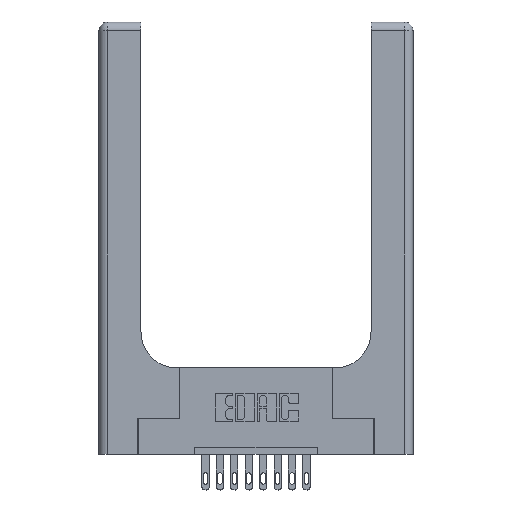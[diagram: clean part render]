
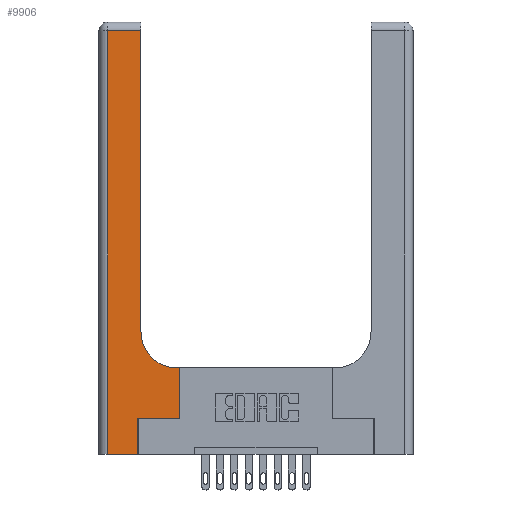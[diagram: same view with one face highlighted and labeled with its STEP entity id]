
A CAD part, top view. The second image highlights one B-rep face of the part: STEP entity #9906.
In plain terms, the highlighted planar face has unit normal (0, 0, 1).
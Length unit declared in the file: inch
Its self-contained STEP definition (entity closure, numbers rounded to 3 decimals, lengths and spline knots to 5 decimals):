
#43 = DIRECTION ( 'NONE',  ( 1., 0., 0. ) ) ;
#279 = LINE ( 'NONE', #14353, #12806 ) ;
#327 = LINE ( 'NONE', #10637, #10549 ) ;
#335 = CARTESIAN_POINT ( 'NONE',  ( 0.269, 0., 0.37 ) ) ;
#378 = CARTESIAN_POINT ( 'NONE',  ( 0.2915, 3., 0.37 ) ) ;
#451 = AXIS2_PLACEMENT_3D ( 'NONE', #11654, #6696, #12667 ) ;
#1412 = ORIENTED_EDGE ( 'NONE', *, *, #4250, .T. ) ;
#1574 = VECTOR ( 'NONE', #10758, 39.37008 ) ;
#1740 = AXIS2_PLACEMENT_3D ( 'NONE', #13222, #12018, #9772 ) ;
#1998 = VERTEX_POINT ( 'NONE', #11737 ) ;
#2088 = CARTESIAN_POINT ( 'NONE',  ( 0.5585, 0.25, 0.37 ) ) ;
#2108 = DIRECTION ( 'NONE',  ( -1., 0., 0. ) ) ;
#2135 = ORIENTED_EDGE ( 'NONE', *, *, #12017, .T. ) ;
#2408 = VERTEX_POINT ( 'NONE', #10790 ) ;
#2549 = FACE_OUTER_BOUND ( 'NONE', #7298, .T. ) ;
#2567 = VERTEX_POINT ( 'NONE', #14894 ) ;
#3411 = DIRECTION ( 'NONE',  ( 1., 0., 0. ) ) ;
#3450 = ORIENTED_EDGE ( 'NONE', *, *, #12003, .T. ) ;
#3453 = CARTESIAN_POINT ( 'NONE',  ( 0., 2.94, 0.37 ) ) ;
#3494 = VECTOR ( 'NONE', #13205, 39.37008 ) ;
#3548 = VERTEX_POINT ( 'NONE', #5660 ) ;
#4115 = VECTOR ( 'NONE', #2108, 39.37008 ) ;
#4157 = CARTESIAN_POINT ( 'NONE',  ( 0.5585, 0.25, 0.37 ) ) ;
#4250 = EDGE_CURVE ( 'NONE', #1998, #5086, #327, .T. ) ;
#4364 = CARTESIAN_POINT ( 'NONE',  ( 0.06, 2.94, 0.37 ) ) ;
#4404 = EDGE_CURVE ( 'NONE', #8872, #10673, #14927, .T. ) ;
#4562 = LINE ( 'NONE', #7578, #6825 ) ;
#5086 = VERTEX_POINT ( 'NONE', #335 ) ;
#5412 = ORIENTED_EDGE ( 'NONE', *, *, #12588, .T. ) ;
#5660 = CARTESIAN_POINT ( 'NONE',  ( 0.2915, 2.94, 0.37 ) ) ;
#5820 = DIRECTION ( 'NONE',  ( 0., 1., 0. ) ) ;
#5900 = CIRCLE ( 'NONE', #451, 0.25 ) ;
#6543 = LINE ( 'NONE', #10487, #4115 ) ;
#6633 = LINE ( 'NONE', #378, #7564 ) ;
#6696 = DIRECTION ( 'NONE',  ( 0., 0., -1. ) ) ;
#6825 = VECTOR ( 'NONE', #7738, 39.37008 ) ;
#7298 = EDGE_LOOP ( 'NONE', ( #9210, #5412, #9057, #1412, #2135, #12947, #3450, #10507, #13886 ) ) ;
#7300 = CARTESIAN_POINT ( 'NONE',  ( 0.269, 0.25, 0.37 ) ) ;
#7464 = EDGE_CURVE ( 'NONE', #11792, #3548, #6633, .T. ) ;
#7564 = VECTOR ( 'NONE', #7796, 39.37008 ) ;
#7578 = CARTESIAN_POINT ( 'NONE',  ( 0.06, 3., 0.37 ) ) ;
#7738 = DIRECTION ( 'NONE',  ( 0., -1., 0. ) ) ;
#7796 = DIRECTION ( 'NONE',  ( 0., 1., 0. ) ) ;
#7916 = EDGE_CURVE ( 'NONE', #8691, #1998, #4562, .T. ) ;
#8691 = VERTEX_POINT ( 'NONE', #4364 ) ;
#8872 = VERTEX_POINT ( 'NONE', #7300 ) ;
#9057 = ORIENTED_EDGE ( 'NONE', *, *, #7916, .T. ) ;
#9210 = ORIENTED_EDGE ( 'NONE', *, *, #7464, .T. ) ;
#9339 = EDGE_CURVE ( 'NONE', #2408, #2567, #6543, .T. ) ;
#9772 = DIRECTION ( 'NONE',  ( -1., 0., 0. ) ) ;
#9906 = ADVANCED_FACE ( 'NONE', ( #2549 ), #11972, .F. ) ;
#10487 = CARTESIAN_POINT ( 'NONE',  ( 0.2915, 0.6, 0.37 ) ) ;
#10507 = ORIENTED_EDGE ( 'NONE', *, *, #9339, .T. ) ;
#10549 = VECTOR ( 'NONE', #43, 39.37008 ) ;
#10637 = CARTESIAN_POINT ( 'NONE',  ( 0., 0., 0.37 ) ) ;
#10664 = LINE ( 'NONE', #3453, #1574 ) ;
#10673 = VERTEX_POINT ( 'NONE', #4157 ) ;
#10758 = DIRECTION ( 'NONE',  ( -1., 0., 0. ) ) ;
#10790 = CARTESIAN_POINT ( 'NONE',  ( 0.5585, 0.6, 0.37 ) ) ;
#11348 = EDGE_CURVE ( 'NONE', #2567, #11792, #5900, .T. ) ;
#11654 = CARTESIAN_POINT ( 'NONE',  ( 0.5415, 0.85, 0.37 ) ) ;
#11737 = CARTESIAN_POINT ( 'NONE',  ( 0.06, 0., 0.37 ) ) ;
#11792 = VERTEX_POINT ( 'NONE', #13587 ) ;
#11972 = PLANE ( 'NONE',  #1740 ) ;
#12003 = EDGE_CURVE ( 'NONE', #10673, #2408, #14508, .T. ) ;
#12017 = EDGE_CURVE ( 'NONE', #5086, #8872, #279, .T. ) ;
#12018 = DIRECTION ( 'NONE',  ( 0., 0., -1. ) ) ;
#12467 = VECTOR ( 'NONE', #3411, 39.37008 ) ;
#12588 = EDGE_CURVE ( 'NONE', #3548, #8691, #10664, .T. ) ;
#12667 = DIRECTION ( 'NONE',  ( 1., 0., 0. ) ) ;
#12806 = VECTOR ( 'NONE', #5820, 39.37008 ) ;
#12947 = ORIENTED_EDGE ( 'NONE', *, *, #4404, .T. ) ;
#13205 = DIRECTION ( 'NONE',  ( 0., 1., 0. ) ) ;
#13222 = CARTESIAN_POINT ( 'NONE',  ( 0., 3., 0.37 ) ) ;
#13587 = CARTESIAN_POINT ( 'NONE',  ( 0.2915, 0.85, 0.37 ) ) ;
#13886 = ORIENTED_EDGE ( 'NONE', *, *, #11348, .T. ) ;
#14254 = CARTESIAN_POINT ( 'NONE',  ( 0.269, 0.25, 0.37 ) ) ;
#14353 = CARTESIAN_POINT ( 'NONE',  ( 0.269, 0., 0.37 ) ) ;
#14508 = LINE ( 'NONE', #2088, #3494 ) ;
#14894 = CARTESIAN_POINT ( 'NONE',  ( 0.5415, 0.6, 0.37 ) ) ;
#14927 = LINE ( 'NONE', #14254, #12467 ) ;
